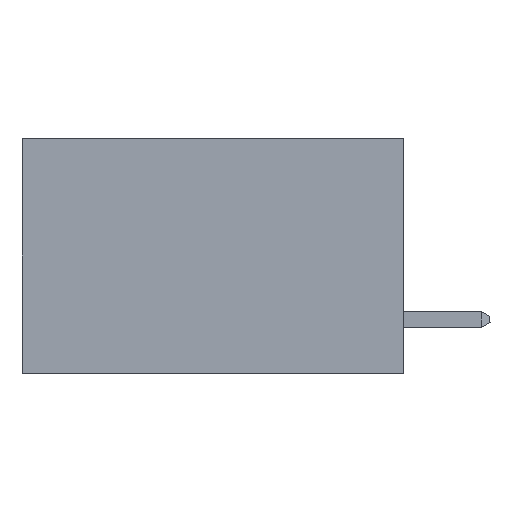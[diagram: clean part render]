
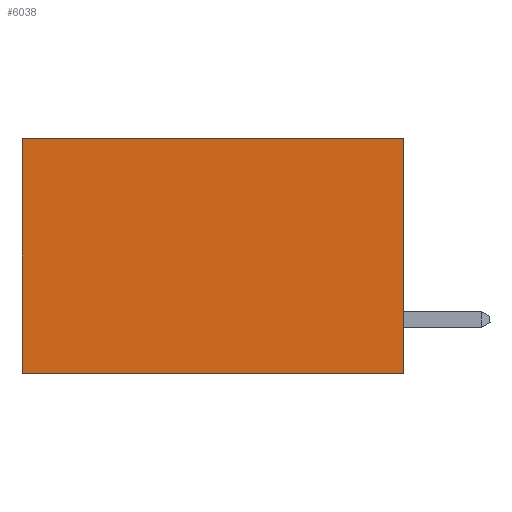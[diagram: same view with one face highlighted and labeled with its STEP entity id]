
A CAD part, left-side view. The second image highlights one B-rep face of the part: STEP entity #6038.
In plain terms, the highlighted planar face has unit normal (-1, 0, 0).
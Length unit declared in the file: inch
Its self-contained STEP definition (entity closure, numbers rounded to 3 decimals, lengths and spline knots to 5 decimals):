
#407 = DIRECTION ( 'NONE',  ( 0., 1., 0. ) ) ;
#3774 = CARTESIAN_POINT ( 'NONE',  ( 0.2875, 0.6, -0.37 ) ) ;
#4295 = LINE ( 'NONE', #10368, #9421 ) ;
#4359 = DIRECTION ( 'NONE',  ( 0., 0., -1. ) ) ;
#4986 = CARTESIAN_POINT ( 'NONE',  ( 0.2875, 0., -0.37 ) ) ;
#5583 = CARTESIAN_POINT ( 'NONE',  ( 0.2875, 0.6, 0. ) ) ;
#6038 = ADVANCED_FACE ( 'NONE', ( #21475 ), #21292, .F. ) ;
#8295 = EDGE_CURVE ( 'NONE', #30213, #15912, #18649, .T. ) ;
#8973 = CARTESIAN_POINT ( 'NONE',  ( 0.2875, 0., 0. ) ) ;
#9421 = VECTOR ( 'NONE', #407, 39.37008 ) ;
#10350 = EDGE_CURVE ( 'NONE', #15778, #22848, #18106, .T. ) ;
#10368 = CARTESIAN_POINT ( 'NONE',  ( 0.2875, 0., -0.37 ) ) ;
#12281 = EDGE_LOOP ( 'NONE', ( #22268, #13806, #19904, #21361 ) ) ;
#12348 = VECTOR ( 'NONE', #15734, 39.37008 ) ;
#13770 = DIRECTION ( 'NONE',  ( 1., 0., 0. ) ) ;
#13806 = ORIENTED_EDGE ( 'NONE', *, *, #22431, .F. ) ;
#15734 = DIRECTION ( 'NONE',  ( 0., 1., 0. ) ) ;
#15778 = VERTEX_POINT ( 'NONE', #5583 ) ;
#15912 = VERTEX_POINT ( 'NONE', #4986 ) ;
#17812 = LINE ( 'NONE', #22813, #12348 ) ;
#18106 = LINE ( 'NONE', #20255, #23143 ) ;
#18649 = LINE ( 'NONE', #8973, #24885 ) ;
#18684 = CARTESIAN_POINT ( 'NONE',  ( 0.2875, 0., 0. ) ) ;
#19904 = ORIENTED_EDGE ( 'NONE', *, *, #8295, .F. ) ;
#20255 = CARTESIAN_POINT ( 'NONE',  ( 0.2875, 0.6, 0. ) ) ;
#20414 = CARTESIAN_POINT ( 'NONE',  ( 0.2875, 0., 0. ) ) ;
#21292 = PLANE ( 'NONE',  #26281 ) ;
#21361 = ORIENTED_EDGE ( 'NONE', *, *, #32497, .T. ) ;
#21475 = FACE_OUTER_BOUND ( 'NONE', #12281, .T. ) ;
#22268 = ORIENTED_EDGE ( 'NONE', *, *, #10350, .T. ) ;
#22431 = EDGE_CURVE ( 'NONE', #15912, #22848, #4295, .T. ) ;
#22813 = CARTESIAN_POINT ( 'NONE',  ( 0.2875, 0., 0. ) ) ;
#22848 = VERTEX_POINT ( 'NONE', #3774 ) ;
#23143 = VECTOR ( 'NONE', #4359, 39.37008 ) ;
#24021 = DIRECTION ( 'NONE',  ( 0., 0., -1. ) ) ;
#24885 = VECTOR ( 'NONE', #28668, 39.37008 ) ;
#26281 = AXIS2_PLACEMENT_3D ( 'NONE', #18684, #13770, #24021 ) ;
#28668 = DIRECTION ( 'NONE',  ( 0., 0., -1. ) ) ;
#30213 = VERTEX_POINT ( 'NONE', #20414 ) ;
#32497 = EDGE_CURVE ( 'NONE', #30213, #15778, #17812, .T. ) ;
